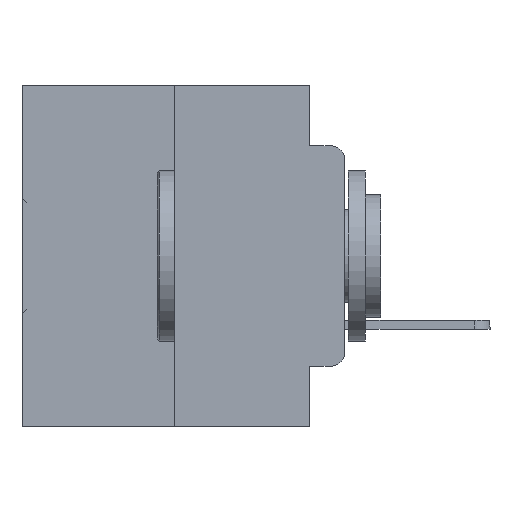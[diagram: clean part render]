
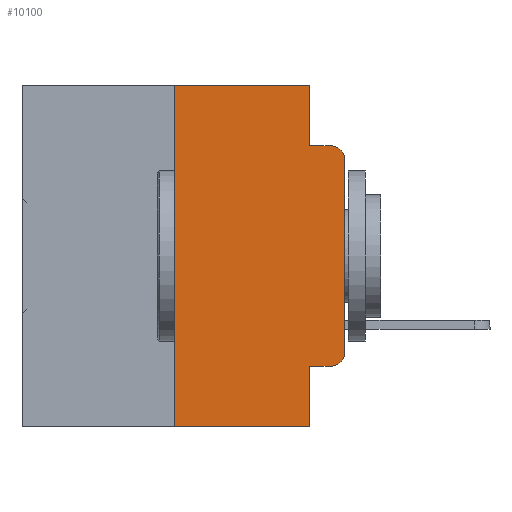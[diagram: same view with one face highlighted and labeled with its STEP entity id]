
A CAD part, left-side view. The second image highlights one B-rep face of the part: STEP entity #10100.
In plain terms, the highlighted planar face has unit normal (-1, 0, 0).
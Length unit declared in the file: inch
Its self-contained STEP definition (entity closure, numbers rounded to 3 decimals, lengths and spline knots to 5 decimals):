
#714 = VERTEX_POINT ( 'NONE', #7632 ) ;
#1453 = DIRECTION ( 'NONE',  ( 0., 0., 1. ) ) ;
#2348 = CARTESIAN_POINT ( 'NONE',  ( 0., 0.051, 0. ) ) ;
#3172 = LINE ( 'NONE', #5872, #31145 ) ;
#3233 = DIRECTION ( 'NONE',  ( 0., -1., 0. ) ) ;
#3313 = DIRECTION ( 'NONE',  ( 0., 0., -1. ) ) ;
#5794 = LINE ( 'NONE', #31959, #11327 ) ;
#5872 = CARTESIAN_POINT ( 'NONE',  ( 0., 0.051, -0.0885 ) ) ;
#6178 = CARTESIAN_POINT ( 'NONE',  ( 0., 0.25, 0. ) ) ;
#6418 = AXIS2_PLACEMENT_3D ( 'NONE', #26449, #16154, #3313 ) ;
#6469 = AXIS2_PLACEMENT_3D ( 'NONE', #8528, #29127, #31986 ) ;
#6838 = VERTEX_POINT ( 'NONE', #14398 ) ;
#7632 = CARTESIAN_POINT ( 'NONE',  ( 0., 0.051, -0.4115 ) ) ;
#8188 = VERTEX_POINT ( 'NONE', #17889 ) ;
#8334 = EDGE_CURVE ( 'NONE', #23354, #28994, #3172, .T. ) ;
#8451 = LINE ( 'NONE', #16050, #18965 ) ;
#8503 = ORIENTED_EDGE ( 'NONE', *, *, #28731, .T. ) ;
#8528 = CARTESIAN_POINT ( 'NONE',  ( 0., 0.02, -0.3915 ) ) ;
#8914 = CARTESIAN_POINT ( 'NONE',  ( 0., 0., -0.1085 ) ) ;
#10008 = ORIENTED_EDGE ( 'NONE', *, *, #17955, .T. ) ;
#10100 = ADVANCED_FACE ( 'NONE', ( #24253 ), #18692, .F. ) ;
#11205 = ORIENTED_EDGE ( 'NONE', *, *, #8334, .F. ) ;
#11327 = VECTOR ( 'NONE', #16106, 39.37008 ) ;
#12366 = EDGE_CURVE ( 'NONE', #21142, #23354, #8451, .T. ) ;
#13543 = LINE ( 'NONE', #13711, #25099 ) ;
#13711 = CARTESIAN_POINT ( 'NONE',  ( 0., 0.473, -0.5 ) ) ;
#14398 = CARTESIAN_POINT ( 'NONE',  ( 0., 0., -0.3915 ) ) ;
#15606 = LINE ( 'NONE', #31460, #21053 ) ;
#15950 = CARTESIAN_POINT ( 'NONE',  ( 0., 0.02, -0.1085 ) ) ;
#15979 = EDGE_CURVE ( 'NONE', #20434, #21774, #33063, .T. ) ;
#16050 = CARTESIAN_POINT ( 'NONE',  ( 0., 0.051, 0. ) ) ;
#16106 = DIRECTION ( 'NONE',  ( 0., 0., -1. ) ) ;
#16154 = DIRECTION ( 'NONE',  ( 1., 0., 0. ) ) ;
#16185 = DIRECTION ( 'NONE',  ( 0., -1., 0. ) ) ;
#16289 = EDGE_CURVE ( 'NONE', #6838, #21365, #27800, .T. ) ;
#16322 = ORIENTED_EDGE ( 'NONE', *, *, #28922, .F. ) ;
#16345 = CIRCLE ( 'NONE', #21226, 0.02 ) ;
#17889 = CARTESIAN_POINT ( 'NONE',  ( 0., 0.051, -0.5 ) ) ;
#17955 = EDGE_CURVE ( 'NONE', #32582, #6838, #21032, .T. ) ;
#18692 = PLANE ( 'NONE',  #6418 ) ;
#18965 = VECTOR ( 'NONE', #20948, 39.37008 ) ;
#19977 = CARTESIAN_POINT ( 'NONE',  ( 0., 0.02, -0.0885 ) ) ;
#20434 = VERTEX_POINT ( 'NONE', #32639 ) ;
#20779 = LINE ( 'NONE', #30897, #28810 ) ;
#20934 = DIRECTION ( 'NONE',  ( 0., -1., 0. ) ) ;
#20948 = DIRECTION ( 'NONE',  ( 0., 0., -1. ) ) ;
#21032 = CIRCLE ( 'NONE', #6469, 0.02 ) ;
#21053 = VECTOR ( 'NONE', #28441, 39.37008 ) ;
#21142 = VERTEX_POINT ( 'NONE', #2348 ) ;
#21226 = AXIS2_PLACEMENT_3D ( 'NONE', #15950, #31302, #28614 ) ;
#21365 = VERTEX_POINT ( 'NONE', #8914 ) ;
#21774 = VERTEX_POINT ( 'NONE', #6178 ) ;
#22235 = CARTESIAN_POINT ( 'NONE',  ( 0., 0., 0. ) ) ;
#22634 = CARTESIAN_POINT ( 'NONE',  ( 0., 0.051, -0.0885 ) ) ;
#23354 = VERTEX_POINT ( 'NONE', #22634 ) ;
#24176 = CARTESIAN_POINT ( 'NONE',  ( 0., 0.02, -0.4115 ) ) ;
#24188 = VECTOR ( 'NONE', #1453, 39.37008 ) ;
#24253 = FACE_OUTER_BOUND ( 'NONE', #33067, .T. ) ;
#24556 = EDGE_CURVE ( 'NONE', #20434, #8188, #13543, .T. ) ;
#24863 = ORIENTED_EDGE ( 'NONE', *, *, #12366, .F. ) ;
#25009 = ORIENTED_EDGE ( 'NONE', *, *, #32010, .T. ) ;
#25099 = VECTOR ( 'NONE', #3233, 39.37008 ) ;
#25319 = VECTOR ( 'NONE', #30691, 39.37008 ) ;
#26440 = ORIENTED_EDGE ( 'NONE', *, *, #32878, .F. ) ;
#26449 = CARTESIAN_POINT ( 'NONE',  ( 0., 0.473, 0. ) ) ;
#27800 = LINE ( 'NONE', #22235, #24188 ) ;
#28257 = ORIENTED_EDGE ( 'NONE', *, *, #16289, .T. ) ;
#28339 = CARTESIAN_POINT ( 'NONE',  ( 0., 0.25, 0. ) ) ;
#28441 = DIRECTION ( 'NONE',  ( 0., -1., 0. ) ) ;
#28614 = DIRECTION ( 'NONE',  ( 0., 0., -1. ) ) ;
#28731 = EDGE_CURVE ( 'NONE', #714, #32582, #15606, .T. ) ;
#28810 = VECTOR ( 'NONE', #20934, 39.37008 ) ;
#28922 = EDGE_CURVE ( 'NONE', #714, #8188, #5794, .T. ) ;
#28994 = VERTEX_POINT ( 'NONE', #19977 ) ;
#29127 = DIRECTION ( 'NONE',  ( -1., 0., 0. ) ) ;
#29737 = ORIENTED_EDGE ( 'NONE', *, *, #15979, .F. ) ;
#30691 = DIRECTION ( 'NONE',  ( 0., 0., 1. ) ) ;
#30897 = CARTESIAN_POINT ( 'NONE',  ( 0., 0.473, 0. ) ) ;
#31093 = ORIENTED_EDGE ( 'NONE', *, *, #24556, .T. ) ;
#31145 = VECTOR ( 'NONE', #16185, 39.37008 ) ;
#31302 = DIRECTION ( 'NONE',  ( -1., 0., 0. ) ) ;
#31460 = CARTESIAN_POINT ( 'NONE',  ( 0., 0.051, -0.4115 ) ) ;
#31959 = CARTESIAN_POINT ( 'NONE',  ( 0., 0.051, 0. ) ) ;
#31986 = DIRECTION ( 'NONE',  ( 0., 0., -1. ) ) ;
#32010 = EDGE_CURVE ( 'NONE', #21365, #28994, #16345, .T. ) ;
#32582 = VERTEX_POINT ( 'NONE', #24176 ) ;
#32639 = CARTESIAN_POINT ( 'NONE',  ( 0., 0.25, -0.5 ) ) ;
#32878 = EDGE_CURVE ( 'NONE', #21774, #21142, #20779, .T. ) ;
#33063 = LINE ( 'NONE', #28339, #25319 ) ;
#33067 = EDGE_LOOP ( 'NONE', ( #28257, #25009, #11205, #24863, #26440, #29737, #31093, #16322, #8503, #10008 ) ) ;
